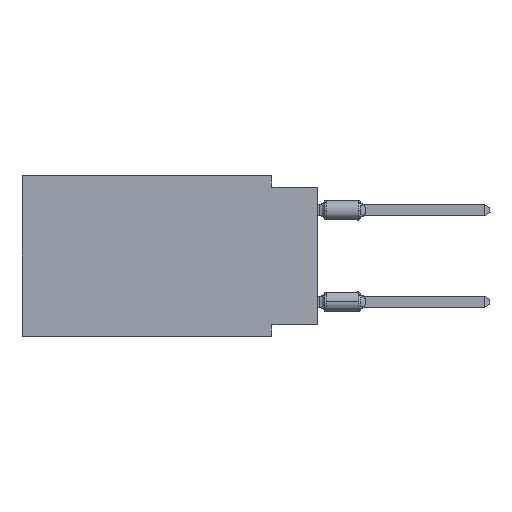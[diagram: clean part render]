
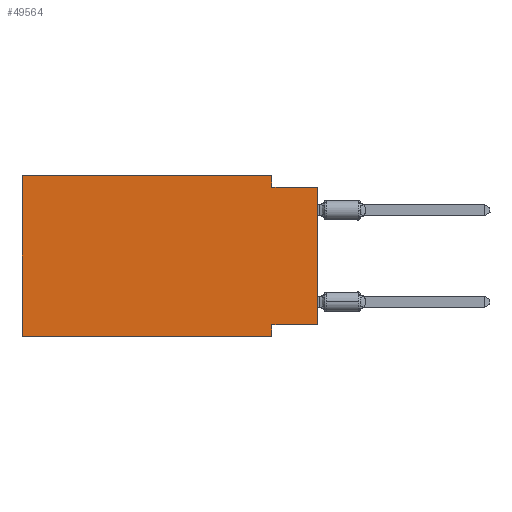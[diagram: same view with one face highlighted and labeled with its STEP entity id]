
A CAD part, left-side view. The second image highlights one B-rep face of the part: STEP entity #49564.
In plain terms, the highlighted planar face has unit normal (-1, 0, 0).
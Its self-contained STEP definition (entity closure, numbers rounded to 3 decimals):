
#66 = EDGE_CURVE ( 'NONE', #26779, #34937, #30156, .T. ) ;
#2347 = LINE ( 'NONE', #69053, #35998 ) ;
#2818 = ORIENTED_EDGE ( 'NONE', *, *, #7334, .T. ) ;
#4115 = VERTEX_POINT ( 'NONE', #46480 ) ;
#4429 = DIRECTION ( 'NONE',  ( 0., 0., 1. ) ) ;
#5404 = LINE ( 'NONE', #62242, #17571 ) ;
#7334 = EDGE_CURVE ( 'NONE', #26779, #33903, #5404, .T. ) ;
#10477 = PLANE ( 'NONE',  #11328 ) ;
#11328 = AXIS2_PLACEMENT_3D ( 'NONE', #55346, #60803, #49507 ) ;
#13252 = CARTESIAN_POINT ( 'NONE',  ( 0., 0., -8.255 ) ) ;
#13971 = DIRECTION ( 'NONE',  ( 0., 1., 0. ) ) ;
#15955 = FACE_OUTER_BOUND ( 'NONE', #60029, .T. ) ;
#17414 = DIRECTION ( 'NONE',  ( 0., -1., 0. ) ) ;
#17571 = VECTOR ( 'NONE', #54988, 1000. ) ;
#17775 = ORIENTED_EDGE ( 'NONE', *, *, #66, .F. ) ;
#18142 = CARTESIAN_POINT ( 'NONE',  ( 0., 2.54, -0.635 ) ) ;
#19300 = CARTESIAN_POINT ( 'NONE',  ( 0., 2.54, 0. ) ) ;
#20712 = EDGE_CURVE ( 'NONE', #24444, #67567, #28916, .T. ) ;
#22391 = DIRECTION ( 'NONE',  ( 0., -1., 0. ) ) ;
#23298 = CARTESIAN_POINT ( 'NONE',  ( 0., 2.54, 0. ) ) ;
#24444 = VERTEX_POINT ( 'NONE', #18142 ) ;
#24668 = CARTESIAN_POINT ( 'NONE',  ( 0., 16.383, 0. ) ) ;
#24723 = DIRECTION ( 'NONE',  ( 0., 0., -1. ) ) ;
#25870 = EDGE_CURVE ( 'NONE', #4115, #67567, #32141, .T. ) ;
#26779 = VERTEX_POINT ( 'NONE', #69087 ) ;
#27815 = ORIENTED_EDGE ( 'NONE', *, *, #25870, .T. ) ;
#27876 = CARTESIAN_POINT ( 'NONE',  ( 0., 0., -0.635 ) ) ;
#27999 = VERTEX_POINT ( 'NONE', #19300 ) ;
#28916 = LINE ( 'NONE', #27876, #69374 ) ;
#29857 = LINE ( 'NONE', #23298, #62462 ) ;
#30156 = LINE ( 'NONE', #24668, #59931 ) ;
#30223 = EDGE_CURVE ( 'NONE', #34937, #27999, #45132, .T. ) ;
#32141 = LINE ( 'NONE', #54388, #38269 ) ;
#33903 = VERTEX_POINT ( 'NONE', #47776 ) ;
#34116 = EDGE_CURVE ( 'NONE', #27999, #24444, #29857, .T. ) ;
#34937 = VERTEX_POINT ( 'NONE', #67597 ) ;
#35341 = ORIENTED_EDGE ( 'NONE', *, *, #47158, .F. ) ;
#35998 = VECTOR ( 'NONE', #63236, 1000. ) ;
#38269 = VECTOR ( 'NONE', #4429, 1000. ) ;
#45132 = LINE ( 'NONE', #67363, #64361 ) ;
#46480 = CARTESIAN_POINT ( 'NONE',  ( 0., 0., -8.255 ) ) ;
#47158 = EDGE_CURVE ( 'NONE', #64736, #33903, #2347, .T. ) ;
#47501 = LINE ( 'NONE', #13252, #58515 ) ;
#47776 = CARTESIAN_POINT ( 'NONE',  ( 0., 2.54, -8.89 ) ) ;
#49507 = DIRECTION ( 'NONE',  ( 0., 0., -1. ) ) ;
#49564 = ADVANCED_FACE ( 'NONE', ( #15955 ), #10477, .F. ) ;
#52356 = CARTESIAN_POINT ( 'NONE',  ( 0., 2.54, -8.255 ) ) ;
#54388 = CARTESIAN_POINT ( 'NONE',  ( 0., 0., 0. ) ) ;
#54496 = ORIENTED_EDGE ( 'NONE', *, *, #20712, .F. ) ;
#54988 = DIRECTION ( 'NONE',  ( 0., -1., 0. ) ) ;
#55346 = CARTESIAN_POINT ( 'NONE',  ( 0., 16.383, 0. ) ) ;
#58515 = VECTOR ( 'NONE', #13971, 1000. ) ;
#59931 = VECTOR ( 'NONE', #69501, 1000. ) ;
#60029 = EDGE_LOOP ( 'NONE', ( #27815, #54496, #67678, #65093, #17775, #2818, #35341, #61775 ) ) ;
#60803 = DIRECTION ( 'NONE',  ( 1., 0., 0. ) ) ;
#61555 = CARTESIAN_POINT ( 'NONE',  ( 0., 0., -0.635 ) ) ;
#61775 = ORIENTED_EDGE ( 'NONE', *, *, #62208, .F. ) ;
#62208 = EDGE_CURVE ( 'NONE', #4115, #64736, #47501, .T. ) ;
#62242 = CARTESIAN_POINT ( 'NONE',  ( 0., 16.383, -8.89 ) ) ;
#62462 = VECTOR ( 'NONE', #24723, 1000. ) ;
#63236 = DIRECTION ( 'NONE',  ( 0., 0., -1. ) ) ;
#64361 = VECTOR ( 'NONE', #17414, 1000. ) ;
#64736 = VERTEX_POINT ( 'NONE', #52356 ) ;
#65093 = ORIENTED_EDGE ( 'NONE', *, *, #30223, .F. ) ;
#67363 = CARTESIAN_POINT ( 'NONE',  ( 0., 16.383, 0. ) ) ;
#67567 = VERTEX_POINT ( 'NONE', #61555 ) ;
#67597 = CARTESIAN_POINT ( 'NONE',  ( 0., 16.383, 0. ) ) ;
#67678 = ORIENTED_EDGE ( 'NONE', *, *, #34116, .F. ) ;
#69053 = CARTESIAN_POINT ( 'NONE',  ( 0., 2.54, -8.89 ) ) ;
#69087 = CARTESIAN_POINT ( 'NONE',  ( 0., 16.383, -8.89 ) ) ;
#69374 = VECTOR ( 'NONE', #22391, 1000. ) ;
#69501 = DIRECTION ( 'NONE',  ( 0., 0., 1. ) ) ;
